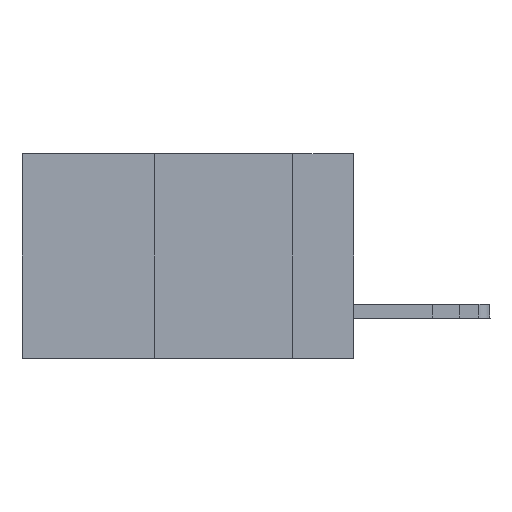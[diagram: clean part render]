
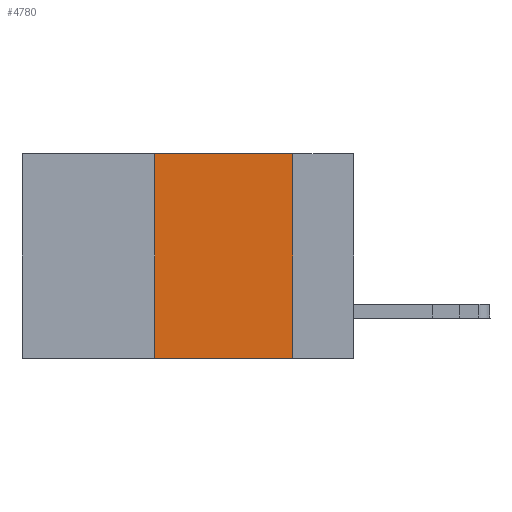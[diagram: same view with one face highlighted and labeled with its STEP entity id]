
A CAD part, left-side view. The second image highlights one B-rep face of the part: STEP entity #4780.
In plain terms, the highlighted planar face has unit normal (-1, 0, 0).
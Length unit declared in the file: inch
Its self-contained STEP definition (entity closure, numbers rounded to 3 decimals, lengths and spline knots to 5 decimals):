
#205 = CARTESIAN_POINT ( 'NONE',  ( 0., 0.11, 0. ) ) ;
#363 = ORIENTED_EDGE ( 'NONE', *, *, #5668, .T. ) ;
#425 = CARTESIAN_POINT ( 'NONE',  ( 0., 0.6, -0.37 ) ) ;
#471 = LINE ( 'NONE', #17905, #8404 ) ;
#1283 = EDGE_LOOP ( 'NONE', ( #16204, #19820, #13358, #363 ) ) ;
#1294 = DIRECTION ( 'NONE',  ( 0., -1., 0. ) ) ;
#1544 = EDGE_CURVE ( 'NONE', #8001, #4617, #471, .T. ) ;
#2626 = CARTESIAN_POINT ( 'NONE',  ( 0., 0.6, 0. ) ) ;
#3444 = VERTEX_POINT ( 'NONE', #205 ) ;
#3838 = DIRECTION ( 'NONE',  ( 0., 0., -1. ) ) ;
#4617 = VERTEX_POINT ( 'NONE', #15655 ) ;
#4780 = ADVANCED_FACE ( 'NONE', ( #12355 ), #11883, .F. ) ;
#5100 = VECTOR ( 'NONE', #1294, 39.37008 ) ;
#5668 = EDGE_CURVE ( 'NONE', #8001, #6426, #10415, .T. ) ;
#6265 = VECTOR ( 'NONE', #3838, 39.37008 ) ;
#6392 = EDGE_CURVE ( 'NONE', #4617, #3444, #17355, .T. ) ;
#6426 = VERTEX_POINT ( 'NONE', #12780 ) ;
#7545 = CARTESIAN_POINT ( 'NONE',  ( 0., 0.6, 0. ) ) ;
#8001 = VERTEX_POINT ( 'NONE', #17671 ) ;
#8404 = VECTOR ( 'NONE', #12083, 39.37008 ) ;
#8824 = DIRECTION ( 'NONE',  ( 0., 0., -1. ) ) ;
#10415 = LINE ( 'NONE', #425, #5100 ) ;
#11561 = CARTESIAN_POINT ( 'NONE',  ( 0., 0.11, 0. ) ) ;
#11883 = PLANE ( 'NONE',  #13364 ) ;
#12083 = DIRECTION ( 'NONE',  ( 0., 0., 1. ) ) ;
#12355 = FACE_OUTER_BOUND ( 'NONE', #1283, .T. ) ;
#12780 = CARTESIAN_POINT ( 'NONE',  ( 0., 0.11, -0.37 ) ) ;
#13068 = VECTOR ( 'NONE', #16789, 39.37008 ) ;
#13314 = LINE ( 'NONE', #11561, #6265 ) ;
#13358 = ORIENTED_EDGE ( 'NONE', *, *, #1544, .F. ) ;
#13364 = AXIS2_PLACEMENT_3D ( 'NONE', #2626, #18027, #8824 ) ;
#15655 = CARTESIAN_POINT ( 'NONE',  ( 0., 0.36, 0. ) ) ;
#16204 = ORIENTED_EDGE ( 'NONE', *, *, #16859, .F. ) ;
#16789 = DIRECTION ( 'NONE',  ( 0., -1., 0. ) ) ;
#16859 = EDGE_CURVE ( 'NONE', #3444, #6426, #13314, .T. ) ;
#17355 = LINE ( 'NONE', #7545, #13068 ) ;
#17671 = CARTESIAN_POINT ( 'NONE',  ( 0., 0.36, -0.37 ) ) ;
#17905 = CARTESIAN_POINT ( 'NONE',  ( 0., 0.36, 0. ) ) ;
#18027 = DIRECTION ( 'NONE',  ( 1., 0., 0. ) ) ;
#19820 = ORIENTED_EDGE ( 'NONE', *, *, #6392, .F. ) ;
